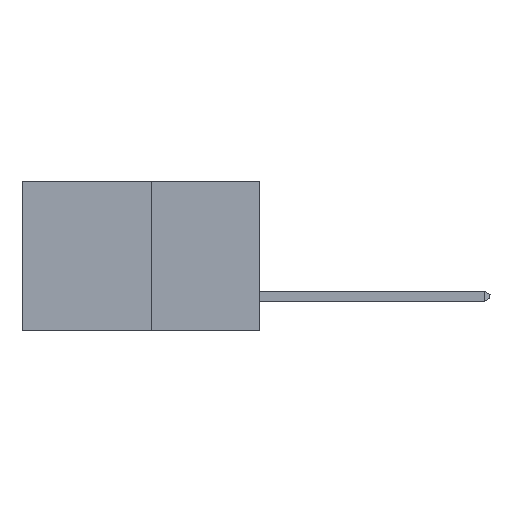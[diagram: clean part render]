
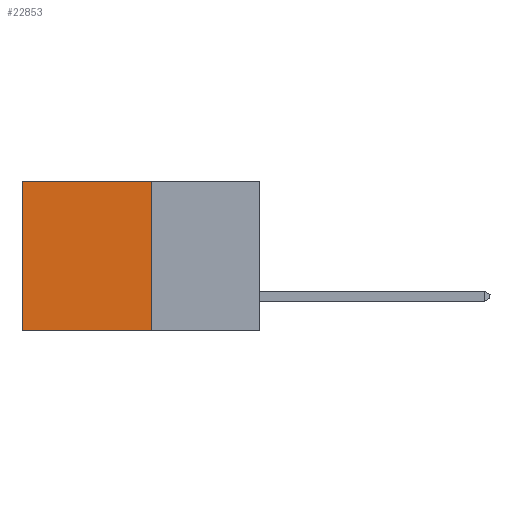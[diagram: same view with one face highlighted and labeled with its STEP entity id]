
A CAD part, left-side view. The second image highlights one B-rep face of the part: STEP entity #22853.
In plain terms, the highlighted planar face has unit normal (-1, 0, 0).
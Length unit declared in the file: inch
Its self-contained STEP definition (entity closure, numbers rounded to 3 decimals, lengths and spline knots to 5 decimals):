
#181 = EDGE_LOOP ( 'NONE', ( #11837, #3613, #13282, #19027 ) ) ;
#542 = VECTOR ( 'NONE', #18205, 39.37008 ) ;
#1991 = CARTESIAN_POINT ( 'NONE',  ( 0.277, 0.27, -0.37 ) ) ;
#2070 = CARTESIAN_POINT ( 'NONE',  ( 0.277, 0.59, -0.37 ) ) ;
#2205 = CARTESIAN_POINT ( 'NONE',  ( 0.277, 0.59, 0. ) ) ;
#3613 = ORIENTED_EDGE ( 'NONE', *, *, #12201, .F. ) ;
#4221 = DIRECTION ( 'NONE',  ( 0., 1., 0. ) ) ;
#5233 = EDGE_CURVE ( 'NONE', #7275, #16801, #6011, .T. ) ;
#5890 = VERTEX_POINT ( 'NONE', #12970 ) ;
#6011 = LINE ( 'NONE', #21555, #10211 ) ;
#7145 = LINE ( 'NONE', #2070, #20742 ) ;
#7272 = DIRECTION ( 'NONE',  ( 0., 0., -1. ) ) ;
#7275 = VERTEX_POINT ( 'NONE', #8956 ) ;
#7352 = VECTOR ( 'NONE', #4221, 39.37008 ) ;
#7488 = VERTEX_POINT ( 'NONE', #2205 ) ;
#8956 = CARTESIAN_POINT ( 'NONE',  ( 0.277, 0.27, 0. ) ) ;
#10211 = VECTOR ( 'NONE', #22834, 39.37008 ) ;
#11031 = DIRECTION ( 'NONE',  ( 0., 0., -1. ) ) ;
#11552 = CARTESIAN_POINT ( 'NONE',  ( 0.277, 0.27, -0.37 ) ) ;
#11837 = ORIENTED_EDGE ( 'NONE', *, *, #18664, .T. ) ;
#12201 = EDGE_CURVE ( 'NONE', #16801, #5890, #19678, .T. ) ;
#12970 = CARTESIAN_POINT ( 'NONE',  ( 0.277, 0.59, -0.37 ) ) ;
#13244 = CARTESIAN_POINT ( 'NONE',  ( 0.277, 0.27, 0. ) ) ;
#13282 = ORIENTED_EDGE ( 'NONE', *, *, #5233, .F. ) ;
#13633 = EDGE_CURVE ( 'NONE', #7275, #7488, #21498, .T. ) ;
#14258 = FACE_OUTER_BOUND ( 'NONE', #181, .T. ) ;
#14449 = CARTESIAN_POINT ( 'NONE',  ( 0.277, 0.27, -0.37 ) ) ;
#16370 = AXIS2_PLACEMENT_3D ( 'NONE', #14449, #17981, #7272 ) ;
#16801 = VERTEX_POINT ( 'NONE', #11552 ) ;
#17407 = PLANE ( 'NONE',  #16370 ) ;
#17981 = DIRECTION ( 'NONE',  ( 1., 0., 0. ) ) ;
#18205 = DIRECTION ( 'NONE',  ( 0., 1., 0. ) ) ;
#18664 = EDGE_CURVE ( 'NONE', #7488, #5890, #7145, .T. ) ;
#19027 = ORIENTED_EDGE ( 'NONE', *, *, #13633, .T. ) ;
#19678 = LINE ( 'NONE', #1991, #542 ) ;
#20742 = VECTOR ( 'NONE', #11031, 39.37008 ) ;
#21498 = LINE ( 'NONE', #13244, #7352 ) ;
#21555 = CARTESIAN_POINT ( 'NONE',  ( 0.277, 0.27, -0.37 ) ) ;
#22834 = DIRECTION ( 'NONE',  ( 0., 0., -1. ) ) ;
#22853 = ADVANCED_FACE ( 'NONE', ( #14258 ), #17407, .F. ) ;
